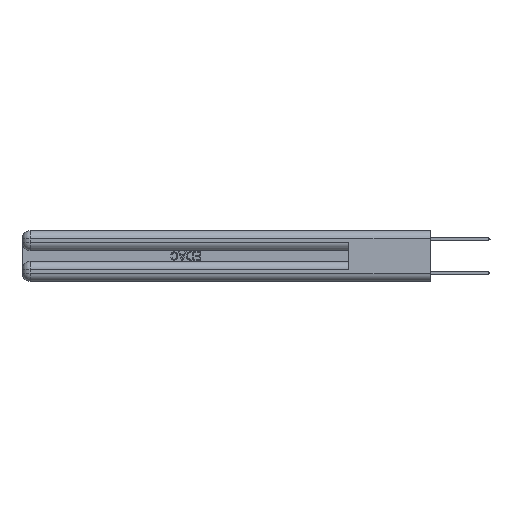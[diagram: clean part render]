
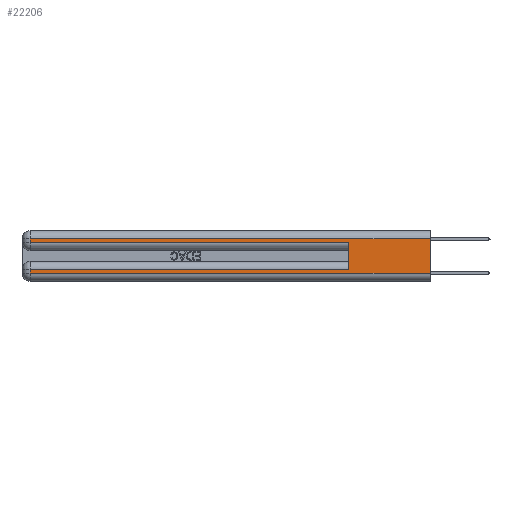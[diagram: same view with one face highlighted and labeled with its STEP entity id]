
A CAD part, left-side view. The second image highlights one B-rep face of the part: STEP entity #22206.
In plain terms, the highlighted planar face has unit normal (-1, 0, 0).
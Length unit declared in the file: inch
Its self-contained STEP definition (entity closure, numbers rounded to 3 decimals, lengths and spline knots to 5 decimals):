
#510 = LINE ( 'NONE', #13863, #30734 ) ;
#594 = EDGE_CURVE ( 'NONE', #1562, #17064, #35162, .T. ) ;
#798 = ORIENTED_EDGE ( 'NONE', *, *, #11168, .F. ) ;
#830 = EDGE_LOOP ( 'NONE', ( #32570, #18758, #12642, #11980, #798, #1489, #31065, #35228 ) ) ;
#1382 = CARTESIAN_POINT ( 'NONE',  ( 0., 2.94, 0.06 ) ) ;
#1489 = ORIENTED_EDGE ( 'NONE', *, *, #594, .T. ) ;
#1562 = VERTEX_POINT ( 'NONE', #29899 ) ;
#1568 = EDGE_CURVE ( 'NONE', #20034, #33336, #510, .T. ) ;
#1848 = DIRECTION ( 'NONE',  ( 1., 0., 0. ) ) ;
#2191 = CARTESIAN_POINT ( 'NONE',  ( 0., 0., 0.37 ) ) ;
#4425 = EDGE_CURVE ( 'NONE', #19788, #20076, #14005, .T. ) ;
#4438 = CARTESIAN_POINT ( 'NONE',  ( 0., 0., 0.37 ) ) ;
#4741 = VECTOR ( 'NONE', #30039, 39.37008 ) ;
#4820 = LINE ( 'NONE', #20695, #24779 ) ;
#5988 = LINE ( 'NONE', #29931, #4741 ) ;
#6266 = LINE ( 'NONE', #12370, #33091 ) ;
#6408 = EDGE_CURVE ( 'NONE', #19788, #19667, #17446, .T. ) ;
#7153 = AXIS2_PLACEMENT_3D ( 'NONE', #2191, #1848, #10309 ) ;
#10309 = DIRECTION ( 'NONE',  ( 0., 0., -1. ) ) ;
#11168 = EDGE_CURVE ( 'NONE', #1562, #33336, #5988, .T. ) ;
#11980 = ORIENTED_EDGE ( 'NONE', *, *, #1568, .T. ) ;
#12370 = CARTESIAN_POINT ( 'NONE',  ( 0., 0., 0.06 ) ) ;
#12577 = CARTESIAN_POINT ( 'NONE',  ( 0., 2.94, 0.285 ) ) ;
#12642 = ORIENTED_EDGE ( 'NONE', *, *, #27362, .T. ) ;
#12889 = DIRECTION ( 'NONE',  ( 0., 0., -1. ) ) ;
#13863 = CARTESIAN_POINT ( 'NONE',  ( 0., 0., 0.285 ) ) ;
#13888 = CARTESIAN_POINT ( 'NONE',  ( 0., 0., 0.31 ) ) ;
#14005 = LINE ( 'NONE', #4438, #31017 ) ;
#15268 = VECTOR ( 'NONE', #19122, 39.37008 ) ;
#15834 = DIRECTION ( 'NONE',  ( 0., -1., 0. ) ) ;
#16002 = EDGE_CURVE ( 'NONE', #31030, #20076, #6266, .T. ) ;
#16633 = CARTESIAN_POINT ( 'NONE',  ( 0., 0.6, 0.285 ) ) ;
#17064 = VERTEX_POINT ( 'NONE', #30098 ) ;
#17446 = LINE ( 'NONE', #22506, #27578 ) ;
#17868 = CARTESIAN_POINT ( 'NONE',  ( 0., 0., 0.085 ) ) ;
#18758 = ORIENTED_EDGE ( 'NONE', *, *, #6408, .T. ) ;
#19122 = DIRECTION ( 'NONE',  ( 0., 0., -1. ) ) ;
#19667 = VERTEX_POINT ( 'NONE', #26710 ) ;
#19788 = VERTEX_POINT ( 'NONE', #13888 ) ;
#19839 = FACE_OUTER_BOUND ( 'NONE', #830, .T. ) ;
#19888 = VECTOR ( 'NONE', #31859, 39.37008 ) ;
#20034 = VERTEX_POINT ( 'NONE', #12577 ) ;
#20076 = VERTEX_POINT ( 'NONE', #20520 ) ;
#20520 = CARTESIAN_POINT ( 'NONE',  ( 0., 0., 0.06 ) ) ;
#20695 = CARTESIAN_POINT ( 'NONE',  ( 0., 2.94, 0.37 ) ) ;
#22206 = ADVANCED_FACE ( 'NONE', ( #19839 ), #29314, .F. ) ;
#22410 = LINE ( 'NONE', #35106, #15268 ) ;
#22506 = CARTESIAN_POINT ( 'NONE',  ( 0., 0., 0.31 ) ) ;
#23084 = DIRECTION ( 'NONE',  ( 0., 0., -1. ) ) ;
#24282 = DIRECTION ( 'NONE',  ( 0., -1., 0. ) ) ;
#24779 = VECTOR ( 'NONE', #12889, 39.37008 ) ;
#26710 = CARTESIAN_POINT ( 'NONE',  ( 0., 2.94, 0.31 ) ) ;
#27362 = EDGE_CURVE ( 'NONE', #19667, #20034, #22410, .T. ) ;
#27578 = VECTOR ( 'NONE', #33711, 39.37008 ) ;
#29128 = EDGE_CURVE ( 'NONE', #17064, #31030, #4820, .T. ) ;
#29314 = PLANE ( 'NONE',  #7153 ) ;
#29899 = CARTESIAN_POINT ( 'NONE',  ( 0., 0.6, 0.085 ) ) ;
#29931 = CARTESIAN_POINT ( 'NONE',  ( 0., 0.6, 0.145 ) ) ;
#30039 = DIRECTION ( 'NONE',  ( 0., 0., 1. ) ) ;
#30098 = CARTESIAN_POINT ( 'NONE',  ( 0., 2.94, 0.085 ) ) ;
#30734 = VECTOR ( 'NONE', #24282, 39.37008 ) ;
#31017 = VECTOR ( 'NONE', #23084, 39.37008 ) ;
#31030 = VERTEX_POINT ( 'NONE', #1382 ) ;
#31065 = ORIENTED_EDGE ( 'NONE', *, *, #29128, .T. ) ;
#31859 = DIRECTION ( 'NONE',  ( 0., 1., 0. ) ) ;
#32570 = ORIENTED_EDGE ( 'NONE', *, *, #4425, .F. ) ;
#33091 = VECTOR ( 'NONE', #15834, 39.37008 ) ;
#33336 = VERTEX_POINT ( 'NONE', #16633 ) ;
#33711 = DIRECTION ( 'NONE',  ( 0., 1., 0. ) ) ;
#35106 = CARTESIAN_POINT ( 'NONE',  ( 0., 2.94, 0.37 ) ) ;
#35162 = LINE ( 'NONE', #17868, #19888 ) ;
#35228 = ORIENTED_EDGE ( 'NONE', *, *, #16002, .T. ) ;
